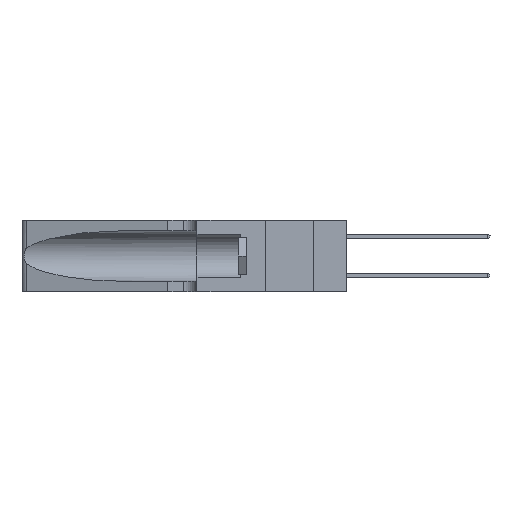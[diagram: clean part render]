
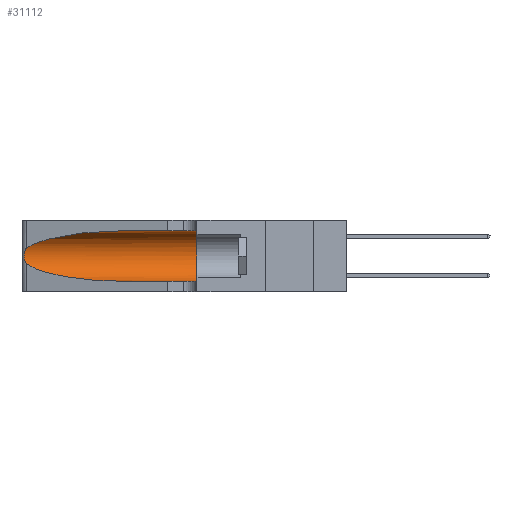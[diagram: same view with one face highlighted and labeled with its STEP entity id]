
A CAD part, left-side view. The second image highlights one B-rep face of the part: STEP entity #31112.
In plain terms, the highlighted cylindrical face has radius 3.308 mm (diameter 6.617 mm), a partial arc.
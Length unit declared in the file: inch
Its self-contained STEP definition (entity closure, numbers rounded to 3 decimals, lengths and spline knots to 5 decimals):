
#1120 = EDGE_LOOP ( 'NONE', ( #5596, #25842, #17572, #28713, #24749, #4807 ) ) ;
#1452 = CARTESIAN_POINT ( 'NONE',  ( 0.26075, 1.23896, 0.178 ) ) ;
#2361 = DIRECTION ( 'NONE',  ( 0., 0., -1. ) ) ;
#2385 = CARTESIAN_POINT ( 'NONE',  ( 0.1305, 0.72297, 0.05475 ) ) ;
#2727 = CARTESIAN_POINT ( 'NONE',  ( 0.1305, 0.72297, 0.05475 ) ) ;
#3180 = VERTEX_POINT ( 'NONE', #14447 ) ;
#3522 = CARTESIAN_POINT ( 'NONE',  ( 0.25487, 1.22718, 0.22369 ) ) ;
#3943 = CARTESIAN_POINT ( 'NONE',  ( 0.25856, 1.23593, 0.16098 ) ) ;
#4561 = VERTEX_POINT ( 'NONE', #2727 ) ;
#4780 = DIRECTION ( 'NONE',  ( 0., -1., 0. ) ) ;
#4807 = ORIENTED_EDGE ( 'NONE', *, *, #11370, .F. ) ;
#5596 = ORIENTED_EDGE ( 'NONE', *, *, #27662, .T. ) ;
#6465 = CARTESIAN_POINT ( 'NONE',  ( 0.25639, 1.23186, 0.15144 ) ) ;
#7516 = CARTESIAN_POINT ( 'NONE',  ( 0.1305, 0.35, 0.05475 ) ) ;
#7664 = VECTOR ( 'NONE', #29524, 39.37008 ) ;
#7869 = EDGE_CURVE ( 'NONE', #29470, #4561, #9628, .T. ) ;
#8924 = CARTESIAN_POINT ( 'NONE',  ( 0.25487, 1.22718, 0.14631 ) ) ;
#8986 = VERTEX_POINT ( 'NONE', #19450 ) ;
#9142 = AXIS2_PLACEMENT_3D ( 'NONE', #27874, #13541, #30265 ) ;
#9628 =( BOUNDED_CURVE ( )  B_SPLINE_CURVE ( 3, ( #28989, #31368, #17069, #2385 ),
 .UNSPECIFIED., .F., .F. ) 
 B_SPLINE_CURVE_WITH_KNOTS ( ( 4, 4 ),
 ( 3.44316, 4.71239 ),
 .UNSPECIFIED. ) 
 CURVE ( )  GEOMETRIC_REPRESENTATION_ITEM ( )  RATIONAL_B_SPLINE_CURVE ( ( 1., 0.87, 0.87, 1. ) ) 
 REPRESENTATION_ITEM ( '' )  );
#9689 = VERTEX_POINT ( 'NONE', #7516 ) ;
#10298 = CARTESIAN_POINT ( 'NONE',  ( 0.1305, 1.61858, 0.05475 ) ) ;
#10914 = CARTESIAN_POINT ( 'NONE',  ( 0.1305, 1.61858, 0.31525 ) ) ;
#11278 = CARTESIAN_POINT ( 'NONE',  ( 0.25639, 1.23184, 0.21858 ) ) ;
#11370 = EDGE_CURVE ( 'NONE', #21011, #3180, #21657, .T. ) ;
#13541 = DIRECTION ( 'NONE',  ( 0., 1., 0. ) ) ;
#13741 = CARTESIAN_POINT ( 'NONE',  ( 0.25854, 1.2359, 0.20912 ) ) ;
#13864 = CYLINDRICAL_SURFACE ( 'NONE', #26733, 0.13025 ) ;
#14447 = CARTESIAN_POINT ( 'NONE',  ( 0.1305, 0.35, 0.31525 ) ) ;
#16128 = CARTESIAN_POINT ( 'NONE',  ( 0.26075, 1.23896, 0.19203 ) ) ;
#16248 =( BOUNDED_CURVE ( )  B_SPLINE_CURVE ( 3, ( #25302, #30078, #18164, #3522 ),
 .UNSPECIFIED., .F., .T. ) 
 B_SPLINE_CURVE_WITH_KNOTS ( ( 4, 4 ),
 ( 1.5708, 2.84003 ),
 .UNSPECIFIED. ) 
 CURVE ( )  GEOMETRIC_REPRESENTATION_ITEM ( )  RATIONAL_B_SPLINE_CURVE ( ( 1., 0.87, 0.87, 1. ) ) 
 REPRESENTATION_ITEM ( '' )  );
#17052 = CARTESIAN_POINT ( 'NONE',  ( 0.1305, 1.61858, 0.185 ) ) ;
#17069 = CARTESIAN_POINT ( 'NONE',  ( 0.18966, 0.96281, 0.05475 ) ) ;
#17196 = EDGE_CURVE ( 'NONE', #4561, #9689, #20549, .T. ) ;
#17572 = ORIENTED_EDGE ( 'NONE', *, *, #7869, .T. ) ;
#18164 = CARTESIAN_POINT ( 'NONE',  ( 0.2373, 1.15595, 0.28018 ) ) ;
#18459 = CARTESIAN_POINT ( 'NONE',  ( 0.25487, 1.22718, 0.22369 ) ) ;
#18566 = CARTESIAN_POINT ( 'NONE',  ( 0.26017, 1.23833, 0.17102 ) ) ;
#18572 = B_SPLINE_CURVE_WITH_KNOTS ( 'NONE', 3,
 ( #18459, #20879, #11278, #28060, #13741, #30461, #16128, #1452, #18566, #3943, #20975, #6465, #23388, #8924 ),
 .UNSPECIFIED., .F., .F.,
 ( 4, 2, 2, 2, 2, 2, 4 ),
 ( 0., 0.00027, 0.00053, 0.00107, 0.0016, 0.00187, 0.00214 ),
 .UNSPECIFIED. ) ;
#19450 = CARTESIAN_POINT ( 'NONE',  ( 0.25487, 1.22718, 0.22369 ) ) ;
#19786 = CARTESIAN_POINT ( 'NONE',  ( 0.25487, 1.22718, 0.14631 ) ) ;
#20549 = LINE ( 'NONE', #10298, #7664 ) ;
#20879 = CARTESIAN_POINT ( 'NONE',  ( 0.25555, 1.22994, 0.2215 ) ) ;
#20975 = CARTESIAN_POINT ( 'NONE',  ( 0.25789, 1.23486, 0.15765 ) ) ;
#21011 = VERTEX_POINT ( 'NONE', #29850 ) ;
#21188 = EDGE_CURVE ( 'NONE', #8986, #29470, #18572, .T. ) ;
#21657 = LINE ( 'NONE', #10914, #27257 ) ;
#23312 = CIRCLE ( 'NONE', #9142, 0.13025 ) ;
#23388 = CARTESIAN_POINT ( 'NONE',  ( 0.25555, 1.22993, 0.14849 ) ) ;
#24749 = ORIENTED_EDGE ( 'NONE', *, *, #30151, .F. ) ;
#25302 = CARTESIAN_POINT ( 'NONE',  ( 0.1305, 0.72297, 0.31525 ) ) ;
#25842 = ORIENTED_EDGE ( 'NONE', *, *, #21188, .T. ) ;
#26599 = FACE_OUTER_BOUND ( 'NONE', #1120, .T. ) ;
#26733 = AXIS2_PLACEMENT_3D ( 'NONE', #17052, #4780, #2361 ) ;
#27257 = VECTOR ( 'NONE', #27704, 39.37008 ) ;
#27662 = EDGE_CURVE ( 'NONE', #21011, #8986, #16248, .T. ) ;
#27704 = DIRECTION ( 'NONE',  ( 0., -1., 0. ) ) ;
#27874 = CARTESIAN_POINT ( 'NONE',  ( 0.1305, 0.35, 0.185 ) ) ;
#28060 = CARTESIAN_POINT ( 'NONE',  ( 0.25787, 1.23484, 0.2124 ) ) ;
#28713 = ORIENTED_EDGE ( 'NONE', *, *, #17196, .T. ) ;
#28989 = CARTESIAN_POINT ( 'NONE',  ( 0.25487, 1.22718, 0.14631 ) ) ;
#29470 = VERTEX_POINT ( 'NONE', #19786 ) ;
#29524 = DIRECTION ( 'NONE',  ( 0., -1., 0. ) ) ;
#29850 = CARTESIAN_POINT ( 'NONE',  ( 0.1305, 0.72297, 0.31525 ) ) ;
#30078 = CARTESIAN_POINT ( 'NONE',  ( 0.18966, 0.96281, 0.31525 ) ) ;
#30151 = EDGE_CURVE ( 'NONE', #3180, #9689, #23312, .T. ) ;
#30265 = DIRECTION ( 'NONE',  ( 0., 0., 1. ) ) ;
#30461 = CARTESIAN_POINT ( 'NONE',  ( 0.26018, 1.23835, 0.19895 ) ) ;
#31112 = ADVANCED_FACE ( 'NONE', ( #26599 ), #13864, .F. ) ;
#31368 = CARTESIAN_POINT ( 'NONE',  ( 0.2373, 1.15595, 0.08982 ) ) ;
